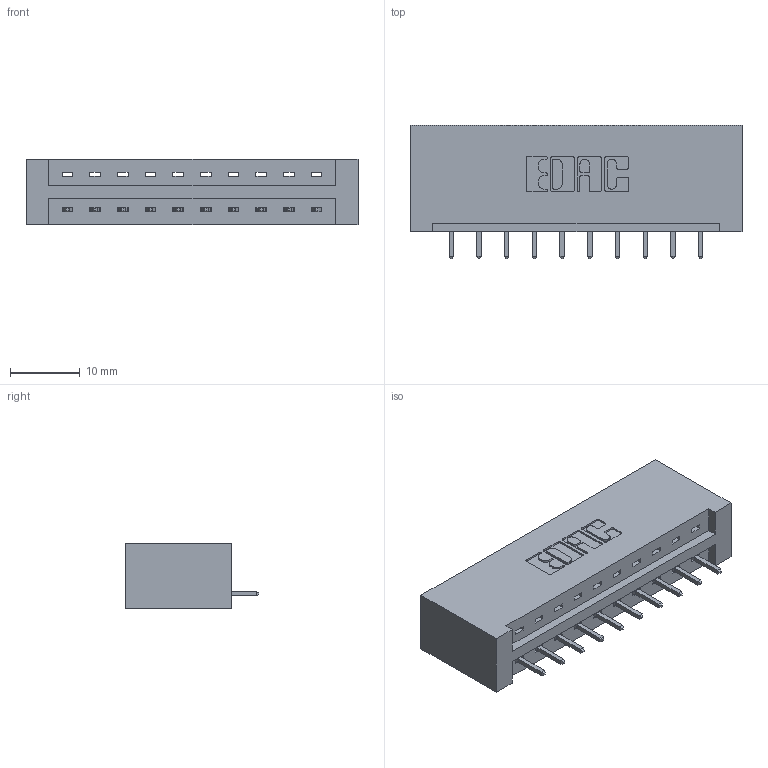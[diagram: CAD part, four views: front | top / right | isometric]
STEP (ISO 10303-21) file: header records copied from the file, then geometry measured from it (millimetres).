
FILE_DESCRIPTION (( 'STEP AP203' ), '1' );
FILE_NAME ('337-010-521-101.STEP', '2018-08-03T23:35:59', ( '' ), ( '' ), 'SwSTEP 2.0', 'SolidWorks 2016', '' );
FILE_SCHEMA (( 'CONFIG_CONTROL_DESIGN' ));
Length unit declared in the file: inch
Products named in the file (3): 345-292-001_345-293-121; 337-010-521-101; 337 Part_No Mounting Lugs
Assembly tree (11 placements, depth 2):
  337-010-521-101
    337 Part_No Mounting Lugs
    345-292-001_345-293-121  x10
Bounding box: 47.5 x 19.06 x 9.4 mm (x, y, z)
Volume: 5246.4 mm3; surface area: 5104.6 mm2
Topology: 11 solids, 11 shells, 726 faces, 2167 edges, 1430 vertices
Faces by surface type: plane 526, cylinder 200
Entity records: 11313 total; most frequent: CARTESIAN_POINT 1976, ORIENTED_EDGE 1922, DIRECTION 1721, EDGE_CURVE 961, LINE 841, VECTOR 841, VERTEX_POINT 638, AXIS2_PLACEMENT_3D 440
